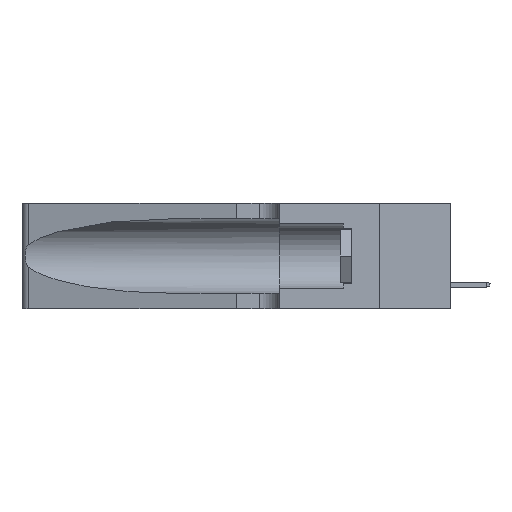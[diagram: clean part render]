
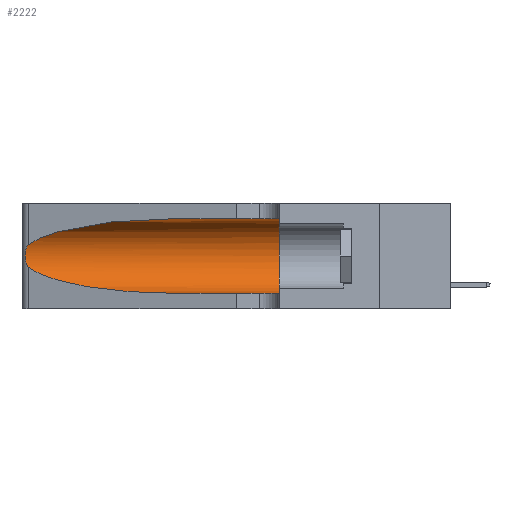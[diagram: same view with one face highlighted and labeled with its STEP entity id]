
A CAD part, left-side view. The second image highlights one B-rep face of the part: STEP entity #2222.
In plain terms, the highlighted cylindrical face has radius 3.308 mm (diameter 6.617 mm), a partial arc.
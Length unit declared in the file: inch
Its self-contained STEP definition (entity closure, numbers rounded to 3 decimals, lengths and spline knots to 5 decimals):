
#65 = CARTESIAN_POINT ( 'NONE',  ( 0.25787, 1.23484, 0.2124 ) ) ;
#140 = EDGE_CURVE ( 'NONE', #15045, #31239, #17929, .T. ) ;
#575 = CARTESIAN_POINT ( 'NONE',  ( 0.25639, 1.23186, 0.15144 ) ) ;
#1737 = VERTEX_POINT ( 'NONE', #17715 ) ;
#1755 = CARTESIAN_POINT ( 'NONE',  ( 0.18966, 0.96281, 0.31525 ) ) ;
#1804 = CARTESIAN_POINT ( 'NONE',  ( 0.25487, 1.22718, 0.14631 ) ) ;
#2050 = DIRECTION ( 'NONE',  ( 0., -1., 0. ) ) ;
#2222 = ADVANCED_FACE ( 'NONE', ( #7039 ), #12700, .F. ) ;
#2381 = DIRECTION ( 'NONE',  ( 0., 0., -1. ) ) ;
#2414 = ORIENTED_EDGE ( 'NONE', *, *, #140, .F. ) ;
#2797 = CARTESIAN_POINT ( 'NONE',  ( 0.26018, 1.23835, 0.19895 ) ) ;
#3710 = CARTESIAN_POINT ( 'NONE',  ( 0.1305, 0.35, 0.31525 ) ) ;
#4782 = CARTESIAN_POINT ( 'NONE',  ( 0.1305, 0.35, 0.185 ) ) ;
#4874 = CARTESIAN_POINT ( 'NONE',  ( 0.1305, 1.61858, 0.31525 ) ) ;
#5547 = CARTESIAN_POINT ( 'NONE',  ( 0.26075, 1.23896, 0.19203 ) ) ;
#5717 = CARTESIAN_POINT ( 'NONE',  ( 0.26075, 1.23896, 0.178 ) ) ;
#6460 = EDGE_CURVE ( 'NONE', #10095, #6663, #26792, .T. ) ;
#6663 = VERTEX_POINT ( 'NONE', #18335 ) ;
#7039 = FACE_OUTER_BOUND ( 'NONE', #26155, .T. ) ;
#7792 = CARTESIAN_POINT ( 'NONE',  ( 0.26017, 1.23833, 0.17102 ) ) ;
#9220 = CARTESIAN_POINT ( 'NONE',  ( 0.18966, 0.96281, 0.05475 ) ) ;
#9952 = ORIENTED_EDGE ( 'NONE', *, *, #12246, .T. ) ;
#10095 = VERTEX_POINT ( 'NONE', #20868 ) ;
#10759 = VECTOR ( 'NONE', #33640, 39.37008 ) ;
#12246 = EDGE_CURVE ( 'NONE', #15045, #1737, #18142, .T. ) ;
#12684 = DIRECTION ( 'NONE',  ( 0., 0., 1. ) ) ;
#12700 = CYLINDRICAL_SURFACE ( 'NONE', #26080, 0.13025 ) ;
#12828 = ORIENTED_EDGE ( 'NONE', *, *, #16348, .T. ) ;
#13454 = CARTESIAN_POINT ( 'NONE',  ( 0.25856, 1.23593, 0.16098 ) ) ;
#14211 = CARTESIAN_POINT ( 'NONE',  ( 0.2373, 1.15595, 0.08982 ) ) ;
#14222 = CARTESIAN_POINT ( 'NONE',  ( 0.25487, 1.22718, 0.14631 ) ) ;
#14758 = EDGE_CURVE ( 'NONE', #28029, #10095, #29933, .T. ) ;
#15045 = VERTEX_POINT ( 'NONE', #18967 ) ;
#16031 = CARTESIAN_POINT ( 'NONE',  ( 0.25487, 1.22718, 0.14631 ) ) ;
#16348 = EDGE_CURVE ( 'NONE', #1737, #28029, #29300, .T. ) ;
#16376 = ORIENTED_EDGE ( 'NONE', *, *, #32175, .F. ) ;
#17104 = CARTESIAN_POINT ( 'NONE',  ( 0.1305, 0.72297, 0.05475 ) ) ;
#17715 = CARTESIAN_POINT ( 'NONE',  ( 0.25487, 1.22718, 0.22369 ) ) ;
#17929 = LINE ( 'NONE', #4874, #10759 ) ;
#18142 =( BOUNDED_CURVE ( )  B_SPLINE_CURVE ( 3, ( #25406, #1755, #33111, #20122 ),
 .UNSPECIFIED., .F., .T. ) 
 B_SPLINE_CURVE_WITH_KNOTS ( ( 4, 4 ),
 ( 1.5708, 2.84003 ),
 .UNSPECIFIED. ) 
 CURVE ( )  GEOMETRIC_REPRESENTATION_ITEM ( )  RATIONAL_B_SPLINE_CURVE ( ( 1., 0.87, 0.87, 1. ) ) 
 REPRESENTATION_ITEM ( '' )  );
#18335 = CARTESIAN_POINT ( 'NONE',  ( 0.1305, 0.35, 0.05475 ) ) ;
#18603 = CARTESIAN_POINT ( 'NONE',  ( 0.25854, 1.2359, 0.20912 ) ) ;
#18894 = AXIS2_PLACEMENT_3D ( 'NONE', #4782, #25684, #12684 ) ;
#18967 = CARTESIAN_POINT ( 'NONE',  ( 0.1305, 0.72297, 0.31525 ) ) ;
#20122 = CARTESIAN_POINT ( 'NONE',  ( 0.25487, 1.22718, 0.22369 ) ) ;
#20570 = CARTESIAN_POINT ( 'NONE',  ( 0.1305, 1.61858, 0.185 ) ) ;
#20833 = VECTOR ( 'NONE', #24211, 39.37008 ) ;
#20868 = CARTESIAN_POINT ( 'NONE',  ( 0.1305, 0.72297, 0.05475 ) ) ;
#20979 = CARTESIAN_POINT ( 'NONE',  ( 0.25789, 1.23486, 0.15765 ) ) ;
#23548 = CARTESIAN_POINT ( 'NONE',  ( 0.25555, 1.22994, 0.2215 ) ) ;
#23891 = CARTESIAN_POINT ( 'NONE',  ( 0.25555, 1.22993, 0.14849 ) ) ;
#24044 = ORIENTED_EDGE ( 'NONE', *, *, #14758, .T. ) ;
#24211 = DIRECTION ( 'NONE',  ( 0., -1., 0. ) ) ;
#25406 = CARTESIAN_POINT ( 'NONE',  ( 0.1305, 0.72297, 0.31525 ) ) ;
#25684 = DIRECTION ( 'NONE',  ( 0., 1., 0. ) ) ;
#25946 = CARTESIAN_POINT ( 'NONE',  ( 0.25487, 1.22718, 0.22369 ) ) ;
#26080 = AXIS2_PLACEMENT_3D ( 'NONE', #20570, #2050, #2381 ) ;
#26155 = EDGE_LOOP ( 'NONE', ( #9952, #12828, #24044, #27799, #16376, #2414 ) ) ;
#26792 = LINE ( 'NONE', #31923, #20833 ) ;
#27799 = ORIENTED_EDGE ( 'NONE', *, *, #6460, .T. ) ;
#28029 = VERTEX_POINT ( 'NONE', #14222 ) ;
#28540 = CARTESIAN_POINT ( 'NONE',  ( 0.25639, 1.23184, 0.21858 ) ) ;
#29300 = B_SPLINE_CURVE_WITH_KNOTS ( 'NONE', 3,
 ( #25946, #23548, #28540, #65, #18603, #2797, #5547, #5717, #7792, #13454, #20979, #575, #23891, #16031 ),
 .UNSPECIFIED., .F., .F.,
 ( 4, 2, 2, 2, 2, 2, 4 ),
 ( 0., 0.00027, 0.00053, 0.00107, 0.0016, 0.00187, 0.00214 ),
 .UNSPECIFIED. ) ;
#29933 =( BOUNDED_CURVE ( )  B_SPLINE_CURVE ( 3, ( #1804, #14211, #9220, #17104 ),
 .UNSPECIFIED., .F., .F. ) 
 B_SPLINE_CURVE_WITH_KNOTS ( ( 4, 4 ),
 ( 3.44316, 4.71239 ),
 .UNSPECIFIED. ) 
 CURVE ( )  GEOMETRIC_REPRESENTATION_ITEM ( )  RATIONAL_B_SPLINE_CURVE ( ( 1., 0.87, 0.87, 1. ) ) 
 REPRESENTATION_ITEM ( '' )  );
#31239 = VERTEX_POINT ( 'NONE', #3710 ) ;
#31923 = CARTESIAN_POINT ( 'NONE',  ( 0.1305, 1.61858, 0.05475 ) ) ;
#32175 = EDGE_CURVE ( 'NONE', #31239, #6663, #33064, .T. ) ;
#33064 = CIRCLE ( 'NONE', #18894, 0.13025 ) ;
#33111 = CARTESIAN_POINT ( 'NONE',  ( 0.2373, 1.15595, 0.28018 ) ) ;
#33640 = DIRECTION ( 'NONE',  ( 0., -1., 0. ) ) ;
